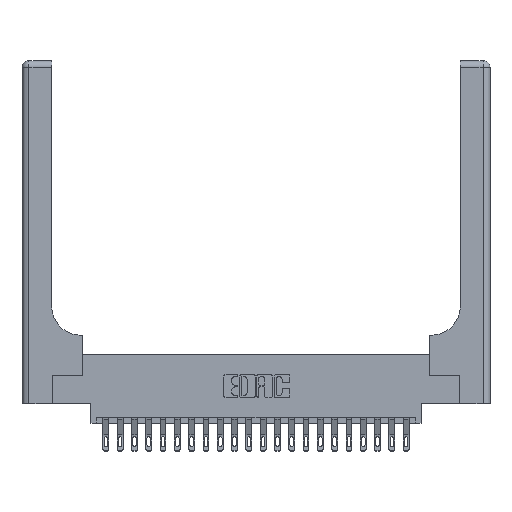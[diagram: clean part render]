
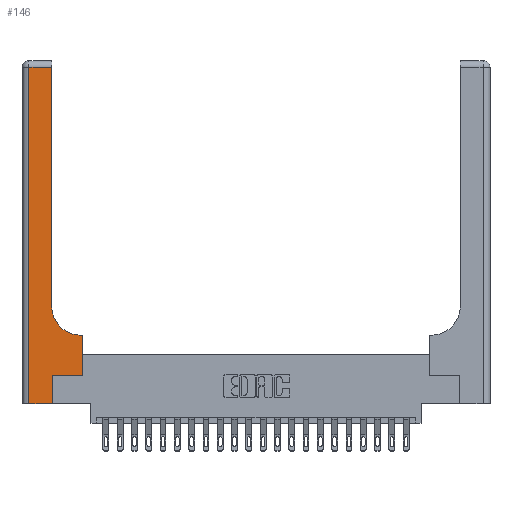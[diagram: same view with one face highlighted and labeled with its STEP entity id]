
A CAD part, top view. The second image highlights one B-rep face of the part: STEP entity #146.
In plain terms, the highlighted planar face has unit normal (0, 0, 1).
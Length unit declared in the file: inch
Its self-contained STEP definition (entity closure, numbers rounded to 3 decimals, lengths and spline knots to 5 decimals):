
#146 = ADVANCED_FACE ( 'NONE', ( #21433 ), #9643, .F. ) ;
#1088 = EDGE_CURVE ( 'NONE', #11935, #6003, #19016, .T. ) ;
#1163 = VERTEX_POINT ( 'NONE', #20483 ) ;
#1256 = VERTEX_POINT ( 'NONE', #6745 ) ;
#1569 = VECTOR ( 'NONE', #19472, 39.37008 ) ;
#1588 = CARTESIAN_POINT ( 'NONE',  ( 0., 2.94, 0.37 ) ) ;
#1698 = EDGE_CURVE ( 'NONE', #9251, #2857, #17456, .T. ) ;
#1882 = CARTESIAN_POINT ( 'NONE',  ( 0.265, 0., 0.37 ) ) ;
#2065 = EDGE_CURVE ( 'NONE', #4777, #11782, #6763, .T. ) ;
#2813 = VECTOR ( 'NONE', #17971, 39.37008 ) ;
#2857 = VERTEX_POINT ( 'NONE', #19750 ) ;
#3120 = EDGE_LOOP ( 'NONE', ( #11171, #3601, #3334, #17009, #12293, #19120, #8622, #10201, #18352 ) ) ;
#3129 = CARTESIAN_POINT ( 'NONE',  ( 0.06, 2.94, 0.37 ) ) ;
#3213 = DIRECTION ( 'NONE',  ( 0., 0., -1. ) ) ;
#3334 = ORIENTED_EDGE ( 'NONE', *, *, #1088, .T. ) ;
#3601 = ORIENTED_EDGE ( 'NONE', *, *, #19297, .T. ) ;
#4308 = EDGE_CURVE ( 'NONE', #1163, #9251, #22172, .T. ) ;
#4475 = CARTESIAN_POINT ( 'NONE',  ( 0.06, 3., 0.37 ) ) ;
#4558 = LINE ( 'NONE', #20589, #17481 ) ;
#4777 = VERTEX_POINT ( 'NONE', #1882 ) ;
#5521 = CARTESIAN_POINT ( 'NONE',  ( 0.265, 0., 0.37 ) ) ;
#5976 = AXIS2_PLACEMENT_3D ( 'NONE', #9640, #21805, #11421 ) ;
#6003 = VERTEX_POINT ( 'NONE', #6838 ) ;
#6745 = CARTESIAN_POINT ( 'NONE',  ( 0.26, 2.94, 0.37 ) ) ;
#6763 = LINE ( 'NONE', #5521, #19088 ) ;
#6838 = CARTESIAN_POINT ( 'NONE',  ( 0.06, 0., 0.37 ) ) ;
#7283 = EDGE_CURVE ( 'NONE', #2857, #1256, #4558, .T. ) ;
#7492 = VECTOR ( 'NONE', #12340, 39.37008 ) ;
#8622 = ORIENTED_EDGE ( 'NONE', *, *, #10210, .T. ) ;
#8737 = EDGE_CURVE ( 'NONE', #11782, #10425, #12239, .T. ) ;
#8986 = CARTESIAN_POINT ( 'NONE',  ( 0., 0., 0.37 ) ) ;
#9080 = DIRECTION ( 'NONE',  ( 0., 1., 0. ) ) ;
#9247 = CARTESIAN_POINT ( 'NONE',  ( 0.528, 0.25, 0.37 ) ) ;
#9251 = VERTEX_POINT ( 'NONE', #22671 ) ;
#9590 = CARTESIAN_POINT ( 'NONE',  ( 0., 3., 0.37 ) ) ;
#9640 = CARTESIAN_POINT ( 'NONE',  ( 0.51, 0.85, 0.37 ) ) ;
#9643 = PLANE ( 'NONE',  #11731 ) ;
#10201 = ORIENTED_EDGE ( 'NONE', *, *, #4308, .T. ) ;
#10210 = EDGE_CURVE ( 'NONE', #10425, #1163, #21389, .T. ) ;
#10425 = VERTEX_POINT ( 'NONE', #9247 ) ;
#10434 = DIRECTION ( 'NONE',  ( -1., 0., 0. ) ) ;
#10467 = LINE ( 'NONE', #1588, #19225 ) ;
#11171 = ORIENTED_EDGE ( 'NONE', *, *, #7283, .T. ) ;
#11421 = DIRECTION ( 'NONE',  ( 1., 0., 0. ) ) ;
#11731 = AXIS2_PLACEMENT_3D ( 'NONE', #9590, #3213, #19341 ) ;
#11782 = VERTEX_POINT ( 'NONE', #16784 ) ;
#11935 = VERTEX_POINT ( 'NONE', #3129 ) ;
#12239 = LINE ( 'NONE', #12726, #2813 ) ;
#12293 = ORIENTED_EDGE ( 'NONE', *, *, #2065, .T. ) ;
#12340 = DIRECTION ( 'NONE',  ( 0., 1., 0. ) ) ;
#12726 = CARTESIAN_POINT ( 'NONE',  ( 0.265, 0.25, 0.37 ) ) ;
#13703 = DIRECTION ( 'NONE',  ( 0., 1., 0. ) ) ;
#13835 = VECTOR ( 'NONE', #18549, 39.37008 ) ;
#15858 = CARTESIAN_POINT ( 'NONE',  ( 0.528, 0.25, 0.37 ) ) ;
#16784 = CARTESIAN_POINT ( 'NONE',  ( 0.265, 0.25, 0.37 ) ) ;
#17009 = ORIENTED_EDGE ( 'NONE', *, *, #21855, .T. ) ;
#17456 = CIRCLE ( 'NONE', #5976, 0.25 ) ;
#17481 = VECTOR ( 'NONE', #13703, 39.37008 ) ;
#17971 = DIRECTION ( 'NONE',  ( 1., 0., 0. ) ) ;
#18172 = VECTOR ( 'NONE', #19897, 39.37008 ) ;
#18352 = ORIENTED_EDGE ( 'NONE', *, *, #1698, .T. ) ;
#18549 = DIRECTION ( 'NONE',  ( 0., -1., 0. ) ) ;
#19016 = LINE ( 'NONE', #4475, #13835 ) ;
#19088 = VECTOR ( 'NONE', #9080, 39.37008 ) ;
#19120 = ORIENTED_EDGE ( 'NONE', *, *, #8737, .T. ) ;
#19225 = VECTOR ( 'NONE', #10434, 39.37008 ) ;
#19297 = EDGE_CURVE ( 'NONE', #1256, #11935, #10467, .T. ) ;
#19341 = DIRECTION ( 'NONE',  ( -1., 0., 0. ) ) ;
#19472 = DIRECTION ( 'NONE',  ( 1., 0., 0. ) ) ;
#19750 = CARTESIAN_POINT ( 'NONE',  ( 0.26, 0.85, 0.37 ) ) ;
#19897 = DIRECTION ( 'NONE',  ( -1., 0., 0. ) ) ;
#20274 = LINE ( 'NONE', #8986, #1569 ) ;
#20483 = CARTESIAN_POINT ( 'NONE',  ( 0.528, 0.6, 0.37 ) ) ;
#20589 = CARTESIAN_POINT ( 'NONE',  ( 0.26, 3., 0.37 ) ) ;
#21389 = LINE ( 'NONE', #15858, #7492 ) ;
#21433 = FACE_OUTER_BOUND ( 'NONE', #3120, .T. ) ;
#21606 = CARTESIAN_POINT ( 'NONE',  ( 0.26, 0.6, 0.37 ) ) ;
#21805 = DIRECTION ( 'NONE',  ( 0., 0., -1. ) ) ;
#21855 = EDGE_CURVE ( 'NONE', #6003, #4777, #20274, .T. ) ;
#22172 = LINE ( 'NONE', #21606, #18172 ) ;
#22671 = CARTESIAN_POINT ( 'NONE',  ( 0.51, 0.6, 0.37 ) ) ;
